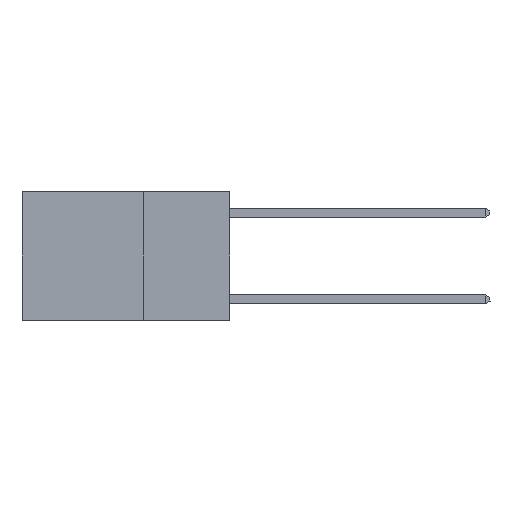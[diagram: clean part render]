
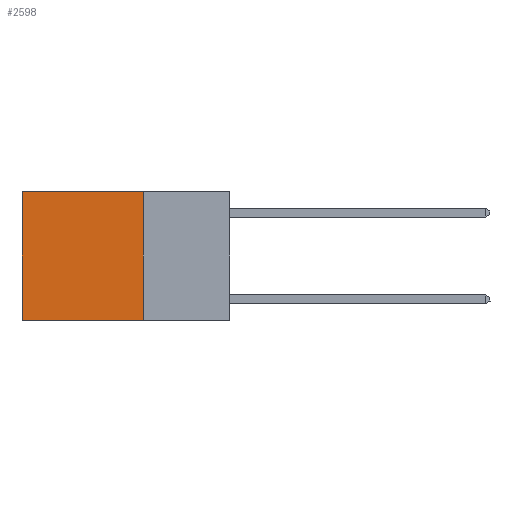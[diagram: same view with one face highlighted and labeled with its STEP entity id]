
A CAD part, left-side view. The second image highlights one B-rep face of the part: STEP entity #2598.
In plain terms, the highlighted planar face has unit normal (-1, 0, 0).
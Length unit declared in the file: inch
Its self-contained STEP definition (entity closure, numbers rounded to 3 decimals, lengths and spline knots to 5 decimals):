
#2598 = ADVANCED_FACE ( 'NONE', ( #21624 ), #12983, .F. ) ;
#2665 = ORIENTED_EDGE ( 'NONE', *, *, #17937, .F. ) ;
#2748 = CARTESIAN_POINT ( 'NONE',  ( 0.2625, 0.25, -0.37 ) ) ;
#3231 = ORIENTED_EDGE ( 'NONE', *, *, #14212, .F. ) ;
#3862 = VECTOR ( 'NONE', #6589, 39.37008 ) ;
#4634 = CARTESIAN_POINT ( 'NONE',  ( 0.2625, 0.6, -0.37 ) ) ;
#5075 = DIRECTION ( 'NONE',  ( 1., 0., 0. ) ) ;
#5865 = EDGE_CURVE ( 'NONE', #22630, #17428, #23427, .T. ) ;
#6589 = DIRECTION ( 'NONE',  ( 0., 1., 0. ) ) ;
#7606 = VERTEX_POINT ( 'NONE', #11051 ) ;
#7727 = CARTESIAN_POINT ( 'NONE',  ( 0.2625, 0.6, 0. ) ) ;
#8620 = CARTESIAN_POINT ( 'NONE',  ( 0.2625, 0.25, 0. ) ) ;
#9200 = VECTOR ( 'NONE', #13605, 39.37008 ) ;
#10000 = DIRECTION ( 'NONE',  ( 0., 0., -1. ) ) ;
#11051 = CARTESIAN_POINT ( 'NONE',  ( 0.2625, 0.25, 0. ) ) ;
#12833 = ORIENTED_EDGE ( 'NONE', *, *, #15161, .T. ) ;
#12983 = PLANE ( 'NONE',  #15101 ) ;
#13605 = DIRECTION ( 'NONE',  ( 0., 0., -1. ) ) ;
#14212 = EDGE_CURVE ( 'NONE', #24036, #17428, #32007, .T. ) ;
#15101 = AXIS2_PLACEMENT_3D ( 'NONE', #25130, #5075, #10000 ) ;
#15161 = EDGE_CURVE ( 'NONE', #7606, #22630, #27193, .T. ) ;
#16235 = CARTESIAN_POINT ( 'NONE',  ( 0.2625, 0.6, 0. ) ) ;
#16438 = DIRECTION ( 'NONE',  ( 0., 0., -1. ) ) ;
#17428 = VERTEX_POINT ( 'NONE', #4634 ) ;
#17937 = EDGE_CURVE ( 'NONE', #7606, #24036, #21055, .T. ) ;
#18245 = VECTOR ( 'NONE', #16438, 39.37008 ) ;
#18919 = CARTESIAN_POINT ( 'NONE',  ( 0.2625, 0.25, 0. ) ) ;
#19179 = CARTESIAN_POINT ( 'NONE',  ( 0.2625, 0.25, -0.37 ) ) ;
#19616 = ORIENTED_EDGE ( 'NONE', *, *, #5865, .T. ) ;
#20073 = VECTOR ( 'NONE', #28678, 39.37008 ) ;
#21055 = LINE ( 'NONE', #8620, #9200 ) ;
#21624 = FACE_OUTER_BOUND ( 'NONE', #30047, .T. ) ;
#22630 = VERTEX_POINT ( 'NONE', #7727 ) ;
#23427 = LINE ( 'NONE', #16235, #18245 ) ;
#24036 = VERTEX_POINT ( 'NONE', #2748 ) ;
#25130 = CARTESIAN_POINT ( 'NONE',  ( 0.2625, 0.25, 0. ) ) ;
#27193 = LINE ( 'NONE', #18919, #20073 ) ;
#28678 = DIRECTION ( 'NONE',  ( 0., 1., 0. ) ) ;
#30047 = EDGE_LOOP ( 'NONE', ( #19616, #3231, #2665, #12833 ) ) ;
#32007 = LINE ( 'NONE', #19179, #3862 ) ;
